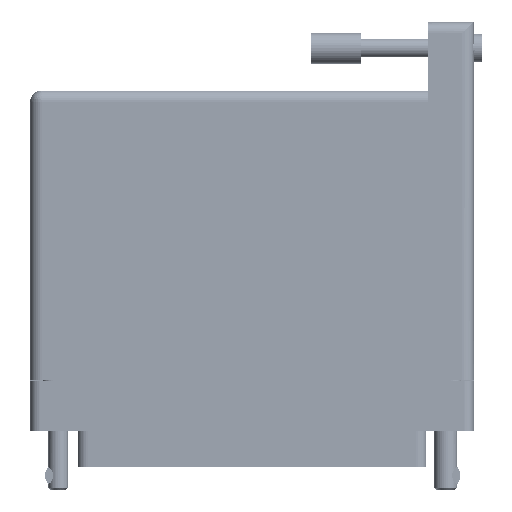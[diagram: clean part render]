
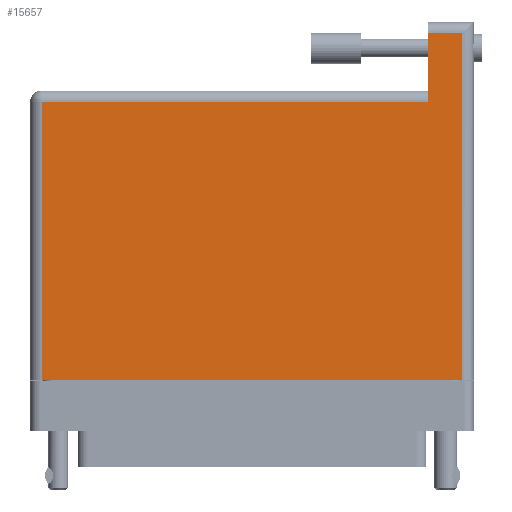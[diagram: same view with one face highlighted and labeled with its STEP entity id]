
A CAD part, front view. The second image highlights one B-rep face of the part: STEP entity #15657.
In plain terms, the highlighted face is planar.
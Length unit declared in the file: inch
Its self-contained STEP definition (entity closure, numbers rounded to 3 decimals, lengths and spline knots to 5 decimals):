
#5222 = LINE ( 'NONE', #64712, #80203 ) ;
#8293 = EDGE_CURVE ( 'NONE', #74702, #19942, #27543, .T. ) ;
#8371 = VECTOR ( 'NONE', #20996, 39.37008 ) ;
#8778 = DIRECTION ( 'NONE',  ( -1., 0., 0. ) ) ;
#12089 = EDGE_LOOP ( 'NONE', ( #45787, #51728, #75710, #48060, #36300, #58024 ) ) ;
#13060 = VECTOR ( 'NONE', #59610, 39.37008 ) ;
#14567 = FACE_OUTER_BOUND ( 'NONE', #12089, .T. ) ;
#15657 = ADVANCED_FACE ( 'NONE', ( #14567 ), #16668, .F. ) ;
#16668 = PLANE ( 'NONE',  #44206 ) ;
#17009 = DIRECTION ( 'NONE',  ( 1., 0., 0. ) ) ;
#18464 = VECTOR ( 'NONE', #57864, 39.37008 ) ;
#19942 = VERTEX_POINT ( 'NONE', #34370 ) ;
#20996 = DIRECTION ( 'NONE',  ( -1., 0., 0. ) ) ;
#23164 = CARTESIAN_POINT ( 'NONE',  ( 1.079, 1.605, 0.617 ) ) ;
#23189 = CARTESIAN_POINT ( 'NONE',  ( -1.359, 1.675, 0.617 ) ) ;
#26928 = CARTESIAN_POINT ( 'NONE',  ( 1.289, 2.025, 0.617 ) ) ;
#27193 = CARTESIAN_POINT ( 'NONE',  ( -1.359, 2.025, 0.617 ) ) ;
#27543 = LINE ( 'NONE', #60944, #66068 ) ;
#29294 = LINE ( 'NONE', #40275, #80955 ) ;
#31755 = CARTESIAN_POINT ( 'NONE',  ( 1.079, 2.095, 0.617 ) ) ;
#32692 = CARTESIAN_POINT ( 'NONE',  ( 1.289, 2.095, 0.617 ) ) ;
#34370 = CARTESIAN_POINT ( 'NONE',  ( -1.289, 1.605, 0.617 ) ) ;
#36300 = ORIENTED_EDGE ( 'NONE', *, *, #82869, .T. ) ;
#40275 = CARTESIAN_POINT ( 'NONE',  ( -1.359, -0.1, 0.617 ) ) ;
#41329 = EDGE_CURVE ( 'NONE', #71880, #58215, #45680, .T. ) ;
#42453 = CARTESIAN_POINT ( 'NONE',  ( 1.079, 2.025, 0.617 ) ) ;
#42787 = DIRECTION ( 'NONE',  ( -1., 0., 0. ) ) ;
#44206 = AXIS2_PLACEMENT_3D ( 'NONE', #23189, #81506, #42787 ) ;
#45187 = CARTESIAN_POINT ( 'NONE',  ( 1.289, -0.1, 0.617 ) ) ;
#45680 = LINE ( 'NONE', #32692, #13060 ) ;
#45787 = ORIENTED_EDGE ( 'NONE', *, *, #8293, .T. ) ;
#46894 = VERTEX_POINT ( 'NONE', #47081 ) ;
#47081 = CARTESIAN_POINT ( 'NONE',  ( -1.289, -0.1, 0.617 ) ) ;
#47297 = EDGE_CURVE ( 'NONE', #51853, #74702, #59923, .T. ) ;
#48060 = ORIENTED_EDGE ( 'NONE', *, *, #41329, .T. ) ;
#48713 = EDGE_CURVE ( 'NONE', #46894, #71880, #29294, .T. ) ;
#51050 = LINE ( 'NONE', #27193, #8371 ) ;
#51728 = ORIENTED_EDGE ( 'NONE', *, *, #61046, .T. ) ;
#51853 = VERTEX_POINT ( 'NONE', #42453 ) ;
#57864 = DIRECTION ( 'NONE',  ( 0., -1., 0. ) ) ;
#58024 = ORIENTED_EDGE ( 'NONE', *, *, #47297, .T. ) ;
#58215 = VERTEX_POINT ( 'NONE', #26928 ) ;
#58453 = DIRECTION ( 'NONE',  ( 0., -1., 0. ) ) ;
#59610 = DIRECTION ( 'NONE',  ( 0., 1., 0. ) ) ;
#59923 = LINE ( 'NONE', #31755, #18464 ) ;
#60944 = CARTESIAN_POINT ( 'NONE',  ( -1.359, 1.605, 0.617 ) ) ;
#61046 = EDGE_CURVE ( 'NONE', #19942, #46894, #5222, .T. ) ;
#64712 = CARTESIAN_POINT ( 'NONE',  ( -1.289, -0.1, 0.617 ) ) ;
#66068 = VECTOR ( 'NONE', #8778, 39.37008 ) ;
#71880 = VERTEX_POINT ( 'NONE', #45187 ) ;
#74702 = VERTEX_POINT ( 'NONE', #23164 ) ;
#75710 = ORIENTED_EDGE ( 'NONE', *, *, #48713, .T. ) ;
#80203 = VECTOR ( 'NONE', #58453, 39.37008 ) ;
#80955 = VECTOR ( 'NONE', #17009, 39.37008 ) ;
#81506 = DIRECTION ( 'NONE',  ( 0., 0., -1. ) ) ;
#82869 = EDGE_CURVE ( 'NONE', #58215, #51853, #51050, .T. ) ;
